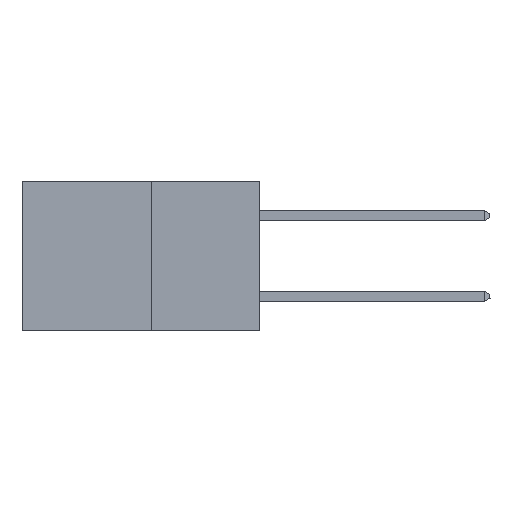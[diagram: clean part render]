
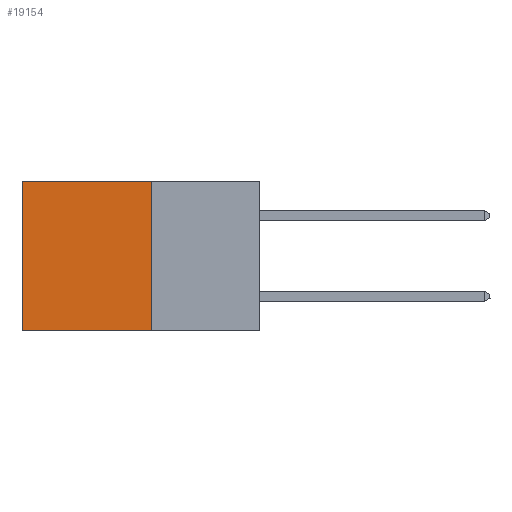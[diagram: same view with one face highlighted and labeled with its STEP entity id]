
A CAD part, left-side view. The second image highlights one B-rep face of the part: STEP entity #19154.
In plain terms, the highlighted planar face has unit normal (-1, 0, 0).
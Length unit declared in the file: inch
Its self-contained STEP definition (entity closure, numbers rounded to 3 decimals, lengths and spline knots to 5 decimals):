
#207 = ORIENTED_EDGE ( 'NONE', *, *, #2896, .F. ) ;
#239 = AXIS2_PLACEMENT_3D ( 'NONE', #13876, #15587, #5322 ) ;
#734 = VERTEX_POINT ( 'NONE', #7826 ) ;
#1853 = EDGE_LOOP ( 'NONE', ( #19934, #2409, #207, #14533 ) ) ;
#1908 = PLANE ( 'NONE',  #239 ) ;
#2409 = ORIENTED_EDGE ( 'NONE', *, *, #11411, .F. ) ;
#2896 = EDGE_CURVE ( 'NONE', #10748, #15789, #13771, .T. ) ;
#3376 = VECTOR ( 'NONE', #5707, 39.37008 ) ;
#5322 = DIRECTION ( 'NONE',  ( 0., 0., -1. ) ) ;
#5707 = DIRECTION ( 'NONE',  ( 0., 1., 0. ) ) ;
#5980 = DIRECTION ( 'NONE',  ( 0., 0., -1. ) ) ;
#6402 = CARTESIAN_POINT ( 'NONE',  ( 0.277, 0.59, -0.37 ) ) ;
#6486 = VECTOR ( 'NONE', #13376, 39.37008 ) ;
#7171 = FACE_OUTER_BOUND ( 'NONE', #1853, .T. ) ;
#7826 = CARTESIAN_POINT ( 'NONE',  ( 0.277, 0.59, 0. ) ) ;
#8072 = VECTOR ( 'NONE', #9507, 39.37008 ) ;
#9507 = DIRECTION ( 'NONE',  ( 0., 0., -1. ) ) ;
#9832 = CARTESIAN_POINT ( 'NONE',  ( 0.277, 0.27, -0.37 ) ) ;
#9961 = VERTEX_POINT ( 'NONE', #6402 ) ;
#10748 = VERTEX_POINT ( 'NONE', #13483 ) ;
#10778 = CARTESIAN_POINT ( 'NONE',  ( 0.277, 0.27, 0. ) ) ;
#11411 = EDGE_CURVE ( 'NONE', #15789, #9961, #15602, .T. ) ;
#11651 = CARTESIAN_POINT ( 'NONE',  ( 0.277, 0.27, -0.37 ) ) ;
#11927 = LINE ( 'NONE', #10778, #3376 ) ;
#12607 = LINE ( 'NONE', #18004, #8072 ) ;
#13376 = DIRECTION ( 'NONE',  ( 0., 1., 0. ) ) ;
#13483 = CARTESIAN_POINT ( 'NONE',  ( 0.277, 0.27, 0. ) ) ;
#13771 = LINE ( 'NONE', #9832, #14315 ) ;
#13876 = CARTESIAN_POINT ( 'NONE',  ( 0.277, 0.27, -0.37 ) ) ;
#14315 = VECTOR ( 'NONE', #5980, 39.37008 ) ;
#14533 = ORIENTED_EDGE ( 'NONE', *, *, #21218, .T. ) ;
#15587 = DIRECTION ( 'NONE',  ( 1., 0., 0. ) ) ;
#15602 = LINE ( 'NONE', #11651, #6486 ) ;
#15789 = VERTEX_POINT ( 'NONE', #16025 ) ;
#16025 = CARTESIAN_POINT ( 'NONE',  ( 0.277, 0.27, -0.37 ) ) ;
#16469 = EDGE_CURVE ( 'NONE', #734, #9961, #12607, .T. ) ;
#18004 = CARTESIAN_POINT ( 'NONE',  ( 0.277, 0.59, -0.37 ) ) ;
#19154 = ADVANCED_FACE ( 'NONE', ( #7171 ), #1908, .F. ) ;
#19934 = ORIENTED_EDGE ( 'NONE', *, *, #16469, .T. ) ;
#21218 = EDGE_CURVE ( 'NONE', #10748, #734, #11927, .T. ) ;
